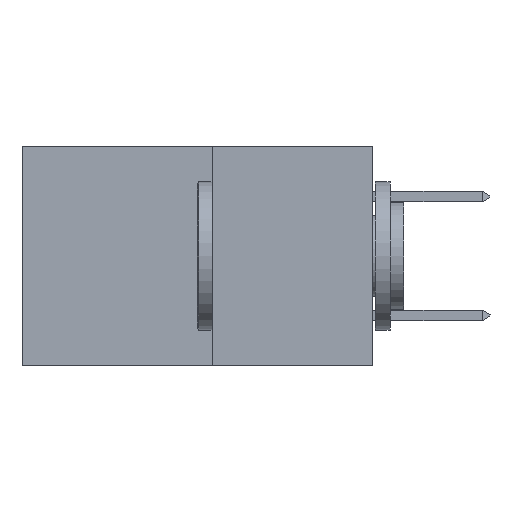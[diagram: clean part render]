
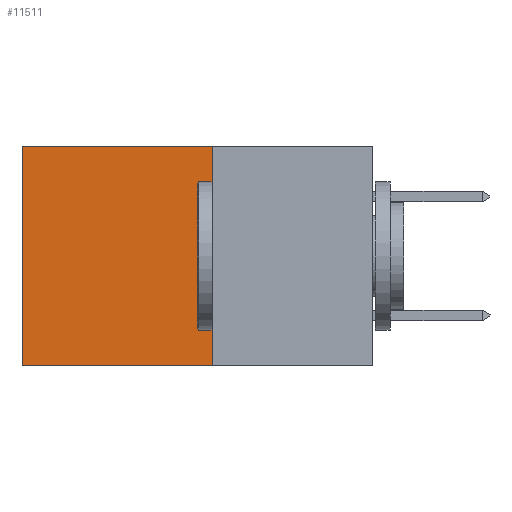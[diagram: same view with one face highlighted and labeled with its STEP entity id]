
A CAD part, left-side view. The second image highlights one B-rep face of the part: STEP entity #11511.
In plain terms, the highlighted planar face has unit normal (-1, 0, 0).
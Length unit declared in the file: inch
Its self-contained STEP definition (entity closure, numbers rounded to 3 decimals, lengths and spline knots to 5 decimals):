
#158 = LINE ( 'NONE', #2917, #20926 ) ;
#358 = CARTESIAN_POINT ( 'NONE',  ( 0.277, 0.59, -0.37 ) ) ;
#634 = FACE_OUTER_BOUND ( 'NONE', #11828, .T. ) ;
#781 = ORIENTED_EDGE ( 'NONE', *, *, #4951, .F. ) ;
#835 = LINE ( 'NONE', #9153, #15250 ) ;
#1332 = VERTEX_POINT ( 'NONE', #17410 ) ;
#1757 = VERTEX_POINT ( 'NONE', #25023 ) ;
#2165 = DIRECTION ( 'NONE',  ( 0., 0., -1. ) ) ;
#2259 = VECTOR ( 'NONE', #6259, 39.37008 ) ;
#2917 = CARTESIAN_POINT ( 'NONE',  ( 0.277, 0.27, 0. ) ) ;
#4951 = EDGE_CURVE ( 'NONE', #1757, #1332, #835, .T. ) ;
#6259 = DIRECTION ( 'NONE',  ( 0., 0., -1. ) ) ;
#6374 = VECTOR ( 'NONE', #8714, 39.37008 ) ;
#8612 = VERTEX_POINT ( 'NONE', #22614 ) ;
#8714 = DIRECTION ( 'NONE',  ( 0., 0., -1. ) ) ;
#9153 = CARTESIAN_POINT ( 'NONE',  ( 0.277, 0.27, -0.37 ) ) ;
#9265 = DIRECTION ( 'NONE',  ( 0., 1., 0. ) ) ;
#9594 = EDGE_CURVE ( 'NONE', #15545, #1332, #12644, .T. ) ;
#11206 = ORIENTED_EDGE ( 'NONE', *, *, #19377, .F. ) ;
#11511 = ADVANCED_FACE ( 'NONE', ( #634 ), #23455, .F. ) ;
#11539 = LINE ( 'NONE', #22237, #6374 ) ;
#11828 = EDGE_LOOP ( 'NONE', ( #15780, #781, #11206, #17596 ) ) ;
#11910 = CARTESIAN_POINT ( 'NONE',  ( 0.277, 0.27, -0.37 ) ) ;
#12554 = AXIS2_PLACEMENT_3D ( 'NONE', #11910, #13878, #2165 ) ;
#12644 = LINE ( 'NONE', #358, #2259 ) ;
#13878 = DIRECTION ( 'NONE',  ( 1., 0., 0. ) ) ;
#14474 = EDGE_CURVE ( 'NONE', #8612, #15545, #158, .T. ) ;
#15250 = VECTOR ( 'NONE', #9265, 39.37008 ) ;
#15545 = VERTEX_POINT ( 'NONE', #24097 ) ;
#15780 = ORIENTED_EDGE ( 'NONE', *, *, #9594, .T. ) ;
#16565 = DIRECTION ( 'NONE',  ( 0., 1., 0. ) ) ;
#17410 = CARTESIAN_POINT ( 'NONE',  ( 0.277, 0.59, -0.37 ) ) ;
#17596 = ORIENTED_EDGE ( 'NONE', *, *, #14474, .T. ) ;
#19377 = EDGE_CURVE ( 'NONE', #8612, #1757, #11539, .T. ) ;
#20926 = VECTOR ( 'NONE', #16565, 39.37008 ) ;
#22237 = CARTESIAN_POINT ( 'NONE',  ( 0.277, 0.27, -0.37 ) ) ;
#22614 = CARTESIAN_POINT ( 'NONE',  ( 0.277, 0.27, 0. ) ) ;
#23455 = PLANE ( 'NONE',  #12554 ) ;
#24097 = CARTESIAN_POINT ( 'NONE',  ( 0.277, 0.59, 0. ) ) ;
#25023 = CARTESIAN_POINT ( 'NONE',  ( 0.277, 0.27, -0.37 ) ) ;
